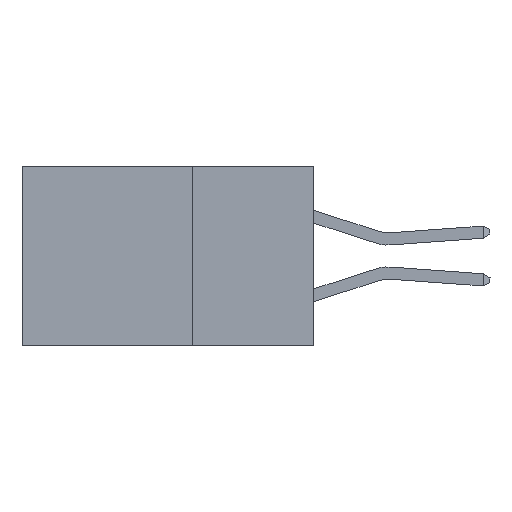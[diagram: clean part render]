
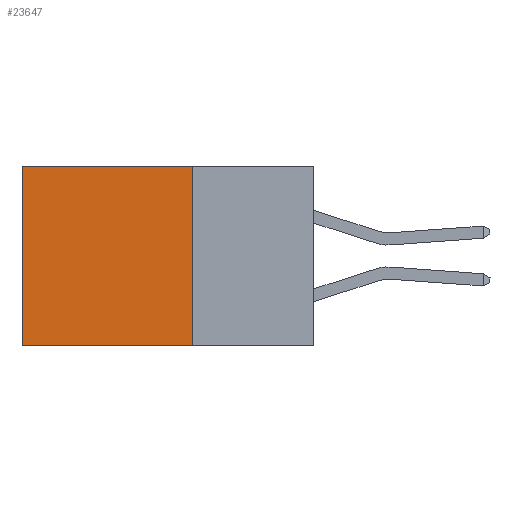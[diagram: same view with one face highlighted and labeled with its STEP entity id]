
A CAD part, left-side view. The second image highlights one B-rep face of the part: STEP entity #23647.
In plain terms, the highlighted planar face has unit normal (-1, 0, 0).
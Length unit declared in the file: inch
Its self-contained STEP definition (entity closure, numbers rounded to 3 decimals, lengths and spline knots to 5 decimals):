
#900 = PLANE ( 'NONE',  #20322 ) ;
#1761 = CARTESIAN_POINT ( 'NONE',  ( 0.2875, 0.25, 0. ) ) ;
#2782 = LINE ( 'NONE', #23424, #24209 ) ;
#2994 = DIRECTION ( 'NONE',  ( 0., 0., -1. ) ) ;
#4124 = EDGE_CURVE ( 'NONE', #28066, #37263, #29701, .T. ) ;
#4517 = ORIENTED_EDGE ( 'NONE', *, *, #4124, .F. ) ;
#5179 = FACE_OUTER_BOUND ( 'NONE', #26164, .T. ) ;
#5317 = LINE ( 'NONE', #30777, #15550 ) ;
#6764 = DIRECTION ( 'NONE',  ( 0., 0., -1. ) ) ;
#7182 = CARTESIAN_POINT ( 'NONE',  ( 0.2875, 0.25, 0. ) ) ;
#8439 = VERTEX_POINT ( 'NONE', #17152 ) ;
#8769 = ORIENTED_EDGE ( 'NONE', *, *, #30148, .T. ) ;
#15550 = VECTOR ( 'NONE', #24325, 39.37008 ) ;
#17152 = CARTESIAN_POINT ( 'NONE',  ( 0.2875, 0.6, -0.37 ) ) ;
#17768 = CARTESIAN_POINT ( 'NONE',  ( 0.2875, 0.6, 0. ) ) ;
#19400 = DIRECTION ( 'NONE',  ( 1., 0., 0. ) ) ;
#20322 = AXIS2_PLACEMENT_3D ( 'NONE', #7182, #19400, #6764 ) ;
#23424 = CARTESIAN_POINT ( 'NONE',  ( 0.2875, 0.6, 0. ) ) ;
#23647 = ADVANCED_FACE ( 'NONE', ( #5179 ), #900, .F. ) ;
#24209 = VECTOR ( 'NONE', #38039, 39.37008 ) ;
#24325 = DIRECTION ( 'NONE',  ( 0., 1., 0. ) ) ;
#26164 = EDGE_LOOP ( 'NONE', ( #8769, #38070, #4517, #37955 ) ) ;
#26947 = EDGE_CURVE ( 'NONE', #37263, #8439, #34517, .T. ) ;
#27595 = CARTESIAN_POINT ( 'NONE',  ( 0.2875, 0.25, 0. ) ) ;
#28066 = VERTEX_POINT ( 'NONE', #1761 ) ;
#28724 = VERTEX_POINT ( 'NONE', #17768 ) ;
#29701 = LINE ( 'NONE', #27595, #39382 ) ;
#30148 = EDGE_CURVE ( 'NONE', #28724, #8439, #2782, .T. ) ;
#30777 = CARTESIAN_POINT ( 'NONE',  ( 0.2875, 0.25, 0. ) ) ;
#30882 = DIRECTION ( 'NONE',  ( 0., 1., 0. ) ) ;
#32602 = VECTOR ( 'NONE', #30882, 39.37008 ) ;
#33970 = CARTESIAN_POINT ( 'NONE',  ( 0.2875, 0.25, -0.37 ) ) ;
#34517 = LINE ( 'NONE', #33970, #32602 ) ;
#37263 = VERTEX_POINT ( 'NONE', #39344 ) ;
#37955 = ORIENTED_EDGE ( 'NONE', *, *, #40171, .T. ) ;
#38039 = DIRECTION ( 'NONE',  ( 0., 0., -1. ) ) ;
#38070 = ORIENTED_EDGE ( 'NONE', *, *, #26947, .F. ) ;
#39344 = CARTESIAN_POINT ( 'NONE',  ( 0.2875, 0.25, -0.37 ) ) ;
#39382 = VECTOR ( 'NONE', #2994, 39.37008 ) ;
#40171 = EDGE_CURVE ( 'NONE', #28066, #28724, #5317, .T. ) ;
